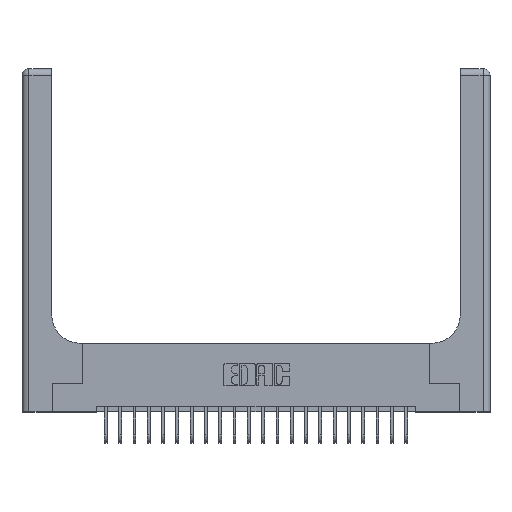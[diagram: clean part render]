
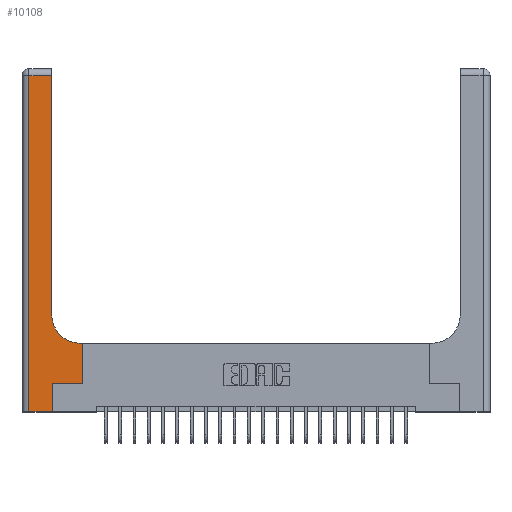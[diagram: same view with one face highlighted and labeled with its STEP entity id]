
A CAD part, top view. The second image highlights one B-rep face of the part: STEP entity #10108.
In plain terms, the highlighted planar face has unit normal (0, 0, 1).
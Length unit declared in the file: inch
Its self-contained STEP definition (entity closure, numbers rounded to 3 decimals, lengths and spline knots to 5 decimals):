
#39 = CARTESIAN_POINT ( 'NONE',  ( 0.265, 0.25, 0.37 ) ) ;
#152 = DIRECTION ( 'NONE',  ( 1., 0., 0. ) ) ;
#352 = CARTESIAN_POINT ( 'NONE',  ( 0.528, 0.6, 0.37 ) ) ;
#569 = DIRECTION ( 'NONE',  ( 0., 1., 0. ) ) ;
#685 = VERTEX_POINT ( 'NONE', #8378 ) ;
#827 = ORIENTED_EDGE ( 'NONE', *, *, #3938, .T. ) ;
#1250 = VECTOR ( 'NONE', #14103, 39.37008 ) ;
#2423 = EDGE_CURVE ( 'NONE', #3011, #14423, #12608, .T. ) ;
#2499 = VECTOR ( 'NONE', #569, 39.37008 ) ;
#2519 = VECTOR ( 'NONE', #7368, 39.37008 ) ;
#2672 = LINE ( 'NONE', #17484, #5261 ) ;
#2691 = ORIENTED_EDGE ( 'NONE', *, *, #16430, .T. ) ;
#2810 = ORIENTED_EDGE ( 'NONE', *, *, #3067, .T. ) ;
#3011 = VERTEX_POINT ( 'NONE', #4005 ) ;
#3067 = EDGE_CURVE ( 'NONE', #10901, #23098, #2672, .T. ) ;
#3938 = EDGE_CURVE ( 'NONE', #15293, #685, #15720, .T. ) ;
#4005 = CARTESIAN_POINT ( 'NONE',  ( 0.528, 0.25, 0.37 ) ) ;
#4687 = EDGE_LOOP ( 'NONE', ( #7177, #2810, #10478, #8452, #2691, #12310, #5370, #21137, #827 ) ) ;
#4835 = VECTOR ( 'NONE', #10202, 39.37008 ) ;
#5261 = VECTOR ( 'NONE', #15378, 39.37008 ) ;
#5305 = VECTOR ( 'NONE', #15963, 39.37008 ) ;
#5370 = ORIENTED_EDGE ( 'NONE', *, *, #2423, .T. ) ;
#5997 = VERTEX_POINT ( 'NONE', #8134 ) ;
#6822 = DIRECTION ( 'NONE',  ( 0., 1., 0. ) ) ;
#7177 = ORIENTED_EDGE ( 'NONE', *, *, #11840, .T. ) ;
#7343 = DIRECTION ( 'NONE',  ( 1., 0., 0. ) ) ;
#7368 = DIRECTION ( 'NONE',  ( 1., 0., 0. ) ) ;
#8134 = CARTESIAN_POINT ( 'NONE',  ( 0.265, 0., 0.37 ) ) ;
#8306 = VECTOR ( 'NONE', #7343, 39.37008 ) ;
#8347 = CARTESIAN_POINT ( 'NONE',  ( 0.528, 0.25, 0.37 ) ) ;
#8378 = CARTESIAN_POINT ( 'NONE',  ( 0.26, 0.85, 0.37 ) ) ;
#8452 = ORIENTED_EDGE ( 'NONE', *, *, #22673, .T. ) ;
#8703 = CARTESIAN_POINT ( 'NONE',  ( 0.06, 2.94, 0.37 ) ) ;
#8909 = PLANE ( 'NONE',  #17194 ) ;
#9284 = CARTESIAN_POINT ( 'NONE',  ( 0.265, 0., 0.37 ) ) ;
#10108 = ADVANCED_FACE ( 'NONE', ( #15935 ), #8909, .F. ) ;
#10202 = DIRECTION ( 'NONE',  ( -1., 0., 0. ) ) ;
#10253 = LINE ( 'NONE', #14263, #1250 ) ;
#10478 = ORIENTED_EDGE ( 'NONE', *, *, #14567, .T. ) ;
#10824 = VECTOR ( 'NONE', #6822, 39.37008 ) ;
#10901 = VERTEX_POINT ( 'NONE', #12647 ) ;
#10921 = LINE ( 'NONE', #22103, #8306 ) ;
#10971 = LINE ( 'NONE', #15877, #4835 ) ;
#11840 = EDGE_CURVE ( 'NONE', #685, #10901, #15580, .T. ) ;
#12310 = ORIENTED_EDGE ( 'NONE', *, *, #23224, .T. ) ;
#12608 = LINE ( 'NONE', #8347, #5305 ) ;
#12634 = DIRECTION ( 'NONE',  ( -1., 0., 0. ) ) ;
#12647 = CARTESIAN_POINT ( 'NONE',  ( 0.26, 2.94, 0.37 ) ) ;
#13046 = CARTESIAN_POINT ( 'NONE',  ( 0., 0., 0.37 ) ) ;
#14103 = DIRECTION ( 'NONE',  ( 0., -1., 0. ) ) ;
#14263 = CARTESIAN_POINT ( 'NONE',  ( 0.06, 3., 0.37 ) ) ;
#14423 = VERTEX_POINT ( 'NONE', #352 ) ;
#14567 = EDGE_CURVE ( 'NONE', #23098, #15473, #10253, .T. ) ;
#15293 = VERTEX_POINT ( 'NONE', #21813 ) ;
#15378 = DIRECTION ( 'NONE',  ( -1., 0., 0. ) ) ;
#15473 = VERTEX_POINT ( 'NONE', #20596 ) ;
#15580 = LINE ( 'NONE', #20930, #2499 ) ;
#15720 = CIRCLE ( 'NONE', #19622, 0.25 ) ;
#15748 = LINE ( 'NONE', #9284, #10824 ) ;
#15877 = CARTESIAN_POINT ( 'NONE',  ( 0.26, 0.6, 0.37 ) ) ;
#15891 = LINE ( 'NONE', #13046, #2519 ) ;
#15935 = FACE_OUTER_BOUND ( 'NONE', #4687, .T. ) ;
#15963 = DIRECTION ( 'NONE',  ( 0., 1., 0. ) ) ;
#16430 = EDGE_CURVE ( 'NONE', #5997, #16513, #15748, .T. ) ;
#16513 = VERTEX_POINT ( 'NONE', #39 ) ;
#17194 = AXIS2_PLACEMENT_3D ( 'NONE', #21886, #23765, #12634 ) ;
#17484 = CARTESIAN_POINT ( 'NONE',  ( 0., 2.94, 0.37 ) ) ;
#18450 = CARTESIAN_POINT ( 'NONE',  ( 0.51, 0.85, 0.37 ) ) ;
#19622 = AXIS2_PLACEMENT_3D ( 'NONE', #18450, #20331, #152 ) ;
#20331 = DIRECTION ( 'NONE',  ( 0., 0., -1. ) ) ;
#20596 = CARTESIAN_POINT ( 'NONE',  ( 0.06, 0., 0.37 ) ) ;
#20930 = CARTESIAN_POINT ( 'NONE',  ( 0.26, 3., 0.37 ) ) ;
#21137 = ORIENTED_EDGE ( 'NONE', *, *, #22402, .T. ) ;
#21813 = CARTESIAN_POINT ( 'NONE',  ( 0.51, 0.6, 0.37 ) ) ;
#21886 = CARTESIAN_POINT ( 'NONE',  ( 0., 3., 0.37 ) ) ;
#22103 = CARTESIAN_POINT ( 'NONE',  ( 0.265, 0.25, 0.37 ) ) ;
#22402 = EDGE_CURVE ( 'NONE', #14423, #15293, #10971, .T. ) ;
#22673 = EDGE_CURVE ( 'NONE', #15473, #5997, #15891, .T. ) ;
#23098 = VERTEX_POINT ( 'NONE', #8703 ) ;
#23224 = EDGE_CURVE ( 'NONE', #16513, #3011, #10921, .T. ) ;
#23765 = DIRECTION ( 'NONE',  ( 0., 0., -1. ) ) ;
